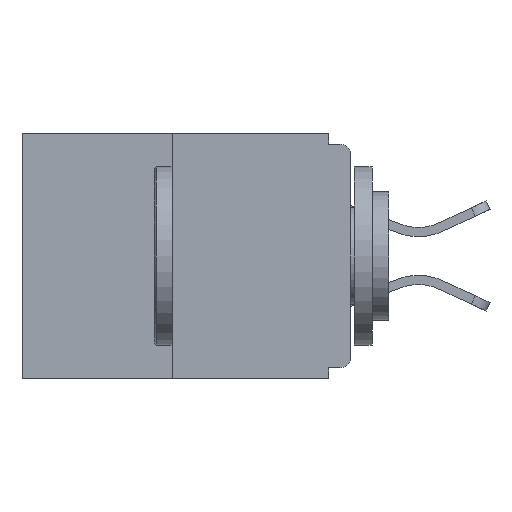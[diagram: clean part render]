
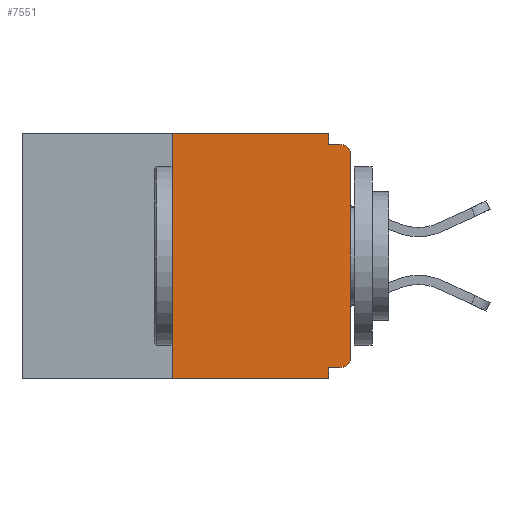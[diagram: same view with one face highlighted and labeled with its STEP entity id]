
A CAD part, left-side view. The second image highlights one B-rep face of the part: STEP entity #7551.
In plain terms, the highlighted planar face has unit normal (-1, 0, 0).
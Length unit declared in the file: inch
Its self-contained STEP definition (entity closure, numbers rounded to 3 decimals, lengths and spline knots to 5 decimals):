
#188 = VECTOR ( 'NONE', #2012, 39.37008 ) ;
#651 = DIRECTION ( 'NONE',  ( 0., 0., -1. ) ) ;
#735 = EDGE_CURVE ( 'NONE', #12822, #6098, #9812, .T. ) ;
#970 = LINE ( 'NONE', #4736, #12406 ) ;
#1047 = VECTOR ( 'NONE', #9722, 39.37008 ) ;
#1101 = LINE ( 'NONE', #2335, #13475 ) ;
#1266 = VECTOR ( 'NONE', #6083, 39.37008 ) ;
#1355 = CARTESIAN_POINT ( 'NONE',  ( 0., 0.031, -0.343 ) ) ;
#1588 = CARTESIAN_POINT ( 'NONE',  ( 0., 0.015, -0.015 ) ) ;
#1710 = CARTESIAN_POINT ( 'NONE',  ( 0., 0., -0.015 ) ) ;
#1788 = DIRECTION ( 'NONE',  ( 0., -1., 0. ) ) ;
#1794 = EDGE_CURVE ( 'NONE', #1840, #2499, #4309, .T. ) ;
#1840 = VERTEX_POINT ( 'NONE', #9283 ) ;
#2012 = DIRECTION ( 'NONE',  ( 0., 1., 0. ) ) ;
#2080 = CARTESIAN_POINT ( 'NONE',  ( 0., 0.015, -0.328 ) ) ;
#2335 = CARTESIAN_POINT ( 'NONE',  ( 0., 0., 0. ) ) ;
#2395 = ORIENTED_EDGE ( 'NONE', *, *, #7794, .T. ) ;
#2499 = VERTEX_POINT ( 'NONE', #4424 ) ;
#2519 = ORIENTED_EDGE ( 'NONE', *, *, #6389, .T. ) ;
#2563 = ORIENTED_EDGE ( 'NONE', *, *, #5730, .F. ) ;
#2694 = CARTESIAN_POINT ( 'NONE',  ( 0., 0.031, -0.015 ) ) ;
#3205 = CARTESIAN_POINT ( 'NONE',  ( 0., 0., -0.328 ) ) ;
#3368 = LINE ( 'NONE', #1710, #1047 ) ;
#3386 = CARTESIAN_POINT ( 'NONE',  ( 0., 0.46, 0. ) ) ;
#3890 = ORIENTED_EDGE ( 'NONE', *, *, #15031, .F. ) ;
#4200 = ORIENTED_EDGE ( 'NONE', *, *, #9096, .F. ) ;
#4309 = LINE ( 'NONE', #9170, #5964 ) ;
#4315 = DIRECTION ( 'NONE',  ( 0., 0., -1. ) ) ;
#4424 = CARTESIAN_POINT ( 'NONE',  ( 0., 0.031, 0. ) ) ;
#4467 = VERTEX_POINT ( 'NONE', #1588 ) ;
#4736 = CARTESIAN_POINT ( 'NONE',  ( 0., 0.25, 0. ) ) ;
#4852 = EDGE_CURVE ( 'NONE', #14413, #1840, #970, .T. ) ;
#5117 = VERTEX_POINT ( 'NONE', #12538 ) ;
#5301 = AXIS2_PLACEMENT_3D ( 'NONE', #12570, #6822, #4315 ) ;
#5416 = DIRECTION ( 'NONE',  ( -1., 0., 0. ) ) ;
#5434 = CARTESIAN_POINT ( 'NONE',  ( 0., 0., -0.313 ) ) ;
#5715 = DIRECTION ( 'NONE',  ( 0., 0., 1. ) ) ;
#5730 = EDGE_CURVE ( 'NONE', #2499, #9013, #6402, .T. ) ;
#5769 = PLANE ( 'NONE',  #11771 ) ;
#5800 = ORIENTED_EDGE ( 'NONE', *, *, #735, .F. ) ;
#5892 = DIRECTION ( 'NONE',  ( 0., 0., 1. ) ) ;
#5964 = VECTOR ( 'NONE', #12665, 39.37008 ) ;
#6083 = DIRECTION ( 'NONE',  ( 0., 0., -1. ) ) ;
#6098 = VERTEX_POINT ( 'NONE', #9617 ) ;
#6185 = EDGE_CURVE ( 'NONE', #12822, #13742, #8532, .T. ) ;
#6389 = EDGE_CURVE ( 'NONE', #13742, #14285, #1101, .T. ) ;
#6402 = LINE ( 'NONE', #14692, #13491 ) ;
#6822 = DIRECTION ( 'NONE',  ( -1., 0., 0. ) ) ;
#7125 = CARTESIAN_POINT ( 'NONE',  ( 0., 0.25, -0.343 ) ) ;
#7206 = ORIENTED_EDGE ( 'NONE', *, *, #4852, .F. ) ;
#7440 = LINE ( 'NONE', #8489, #12365 ) ;
#7523 = EDGE_LOOP ( 'NONE', ( #10198, #7206, #2395, #3890, #5800, #9448, #2519, #9126, #4200, #2563 ) ) ;
#7551 = ADVANCED_FACE ( 'NONE', ( #13270 ), #5769, .F. ) ;
#7794 = EDGE_CURVE ( 'NONE', #14413, #5117, #7440, .T. ) ;
#8489 = CARTESIAN_POINT ( 'NONE',  ( 0., 0.46, -0.343 ) ) ;
#8532 = CIRCLE ( 'NONE', #10185, 0.015 ) ;
#9013 = VERTEX_POINT ( 'NONE', #2694 ) ;
#9096 = EDGE_CURVE ( 'NONE', #9013, #4467, #3368, .T. ) ;
#9126 = ORIENTED_EDGE ( 'NONE', *, *, #12648, .T. ) ;
#9135 = DIRECTION ( 'NONE',  ( 0., 0., -1. ) ) ;
#9170 = CARTESIAN_POINT ( 'NONE',  ( 0., 0.46, 0. ) ) ;
#9283 = CARTESIAN_POINT ( 'NONE',  ( 0., 0.25, 0. ) ) ;
#9448 = ORIENTED_EDGE ( 'NONE', *, *, #6185, .T. ) ;
#9617 = CARTESIAN_POINT ( 'NONE',  ( 0., 0.031, -0.328 ) ) ;
#9722 = DIRECTION ( 'NONE',  ( 0., -1., 0. ) ) ;
#9812 = LINE ( 'NONE', #3205, #188 ) ;
#9925 = DIRECTION ( 'NONE',  ( 0., 0., -1. ) ) ;
#10185 = AXIS2_PLACEMENT_3D ( 'NONE', #14580, #5416, #9925 ) ;
#10198 = ORIENTED_EDGE ( 'NONE', *, *, #1794, .F. ) ;
#10424 = DIRECTION ( 'NONE',  ( 1., 0., 0. ) ) ;
#11771 = AXIS2_PLACEMENT_3D ( 'NONE', #3386, #10424, #9135 ) ;
#12365 = VECTOR ( 'NONE', #1788, 39.37008 ) ;
#12406 = VECTOR ( 'NONE', #5892, 39.37008 ) ;
#12433 = CARTESIAN_POINT ( 'NONE',  ( 0., 0., -0.03 ) ) ;
#12538 = CARTESIAN_POINT ( 'NONE',  ( 0., 0.031, -0.343 ) ) ;
#12552 = LINE ( 'NONE', #1355, #1266 ) ;
#12570 = CARTESIAN_POINT ( 'NONE',  ( 0., 0.015, -0.03 ) ) ;
#12648 = EDGE_CURVE ( 'NONE', #14285, #4467, #13127, .T. ) ;
#12665 = DIRECTION ( 'NONE',  ( 0., -1., 0. ) ) ;
#12822 = VERTEX_POINT ( 'NONE', #2080 ) ;
#13127 = CIRCLE ( 'NONE', #5301, 0.015 ) ;
#13270 = FACE_OUTER_BOUND ( 'NONE', #7523, .T. ) ;
#13475 = VECTOR ( 'NONE', #5715, 39.37008 ) ;
#13491 = VECTOR ( 'NONE', #651, 39.37008 ) ;
#13742 = VERTEX_POINT ( 'NONE', #5434 ) ;
#14285 = VERTEX_POINT ( 'NONE', #12433 ) ;
#14413 = VERTEX_POINT ( 'NONE', #7125 ) ;
#14580 = CARTESIAN_POINT ( 'NONE',  ( 0., 0.015, -0.313 ) ) ;
#14692 = CARTESIAN_POINT ( 'NONE',  ( 0., 0.031, 0. ) ) ;
#15031 = EDGE_CURVE ( 'NONE', #6098, #5117, #12552, .T. ) ;
